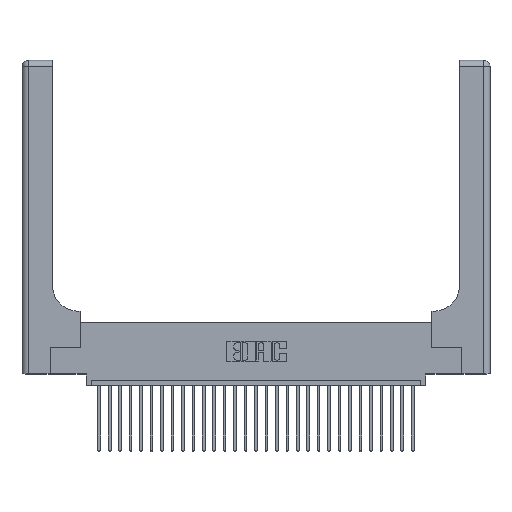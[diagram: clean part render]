
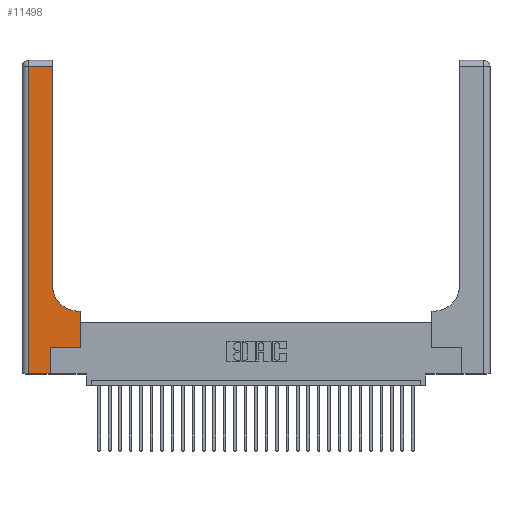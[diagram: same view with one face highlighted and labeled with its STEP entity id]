
A CAD part, top view. The second image highlights one B-rep face of the part: STEP entity #11498.
In plain terms, the highlighted planar face has unit normal (0, 0, 1).
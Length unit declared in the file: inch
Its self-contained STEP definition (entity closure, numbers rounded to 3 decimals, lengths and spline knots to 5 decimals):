
#89 = CARTESIAN_POINT ( 'NONE',  ( 0.5415, 0.6, 0.37 ) ) ;
#427 = CARTESIAN_POINT ( 'NONE',  ( 0.06, 3., 0.37 ) ) ;
#664 = LINE ( 'NONE', #8001, #13792 ) ;
#753 = LINE ( 'NONE', #427, #4031 ) ;
#1092 = DIRECTION ( 'NONE',  ( 1., 0., 0. ) ) ;
#1277 = VERTEX_POINT ( 'NONE', #27150 ) ;
#1534 = CARTESIAN_POINT ( 'NONE',  ( 0., 0., 0.37 ) ) ;
#1841 = DIRECTION ( 'NONE',  ( 1., 0., 0. ) ) ;
#2585 = DIRECTION ( 'NONE',  ( -1., 0., 0. ) ) ;
#2688 = CARTESIAN_POINT ( 'NONE',  ( 0., 3., 0.37 ) ) ;
#2798 = DIRECTION ( 'NONE',  ( 0., -1., 0. ) ) ;
#4031 = VECTOR ( 'NONE', #2798, 39.37008 ) ;
#4500 = CARTESIAN_POINT ( 'NONE',  ( 0., 2.94, 0.37 ) ) ;
#4639 = ORIENTED_EDGE ( 'NONE', *, *, #14295, .T. ) ;
#5188 = CARTESIAN_POINT ( 'NONE',  ( 0.2915, 3., 0.37 ) ) ;
#5705 = VERTEX_POINT ( 'NONE', #14656 ) ;
#5774 = FACE_OUTER_BOUND ( 'NONE', #26763, .T. ) ;
#5904 = VECTOR ( 'NONE', #29011, 39.37008 ) ;
#6970 = VECTOR ( 'NONE', #22443, 39.37008 ) ;
#7249 = CARTESIAN_POINT ( 'NONE',  ( 0.269, 0.25, 0.37 ) ) ;
#7587 = ORIENTED_EDGE ( 'NONE', *, *, #23187, .T. ) ;
#7790 = DIRECTION ( 'NONE',  ( 0., 1., 0. ) ) ;
#8001 = CARTESIAN_POINT ( 'NONE',  ( 0.5585, 0.25, 0.37 ) ) ;
#8144 = EDGE_CURVE ( 'NONE', #1277, #19769, #18276, .T. ) ;
#9527 = ORIENTED_EDGE ( 'NONE', *, *, #21666, .T. ) ;
#9698 = DIRECTION ( 'NONE',  ( 0., 0., -1. ) ) ;
#10090 = CIRCLE ( 'NONE', #21996, 0.25 ) ;
#10268 = LINE ( 'NONE', #26581, #5904 ) ;
#11498 = ADVANCED_FACE ( 'NONE', ( #5774 ), #18615, .F. ) ;
#11927 = DIRECTION ( 'NONE',  ( -1., 0., 0. ) ) ;
#12218 = EDGE_CURVE ( 'NONE', #16540, #15995, #20226, .T. ) ;
#13783 = EDGE_CURVE ( 'NONE', #5705, #16540, #10268, .T. ) ;
#13792 = VECTOR ( 'NONE', #7790, 39.37008 ) ;
#14163 = VECTOR ( 'NONE', #20651, 39.37008 ) ;
#14295 = EDGE_CURVE ( 'NONE', #17094, #5705, #20736, .T. ) ;
#14656 = CARTESIAN_POINT ( 'NONE',  ( 0.269, 0., 0.37 ) ) ;
#14816 = DIRECTION ( 'NONE',  ( 0., 1., 0. ) ) ;
#15369 = ORIENTED_EDGE ( 'NONE', *, *, #15416, .T. ) ;
#15416 = EDGE_CURVE ( 'NONE', #15532, #16965, #28680, .T. ) ;
#15532 = VERTEX_POINT ( 'NONE', #27781 ) ;
#15880 = VECTOR ( 'NONE', #1841, 39.37008 ) ;
#15995 = VERTEX_POINT ( 'NONE', #27072 ) ;
#16064 = ORIENTED_EDGE ( 'NONE', *, *, #13783, .T. ) ;
#16113 = AXIS2_PLACEMENT_3D ( 'NONE', #2688, #9698, #2585 ) ;
#16540 = VERTEX_POINT ( 'NONE', #7249 ) ;
#16965 = VERTEX_POINT ( 'NONE', #89 ) ;
#16997 = ORIENTED_EDGE ( 'NONE', *, *, #27641, .T. ) ;
#17094 = VERTEX_POINT ( 'NONE', #28500 ) ;
#17261 = VERTEX_POINT ( 'NONE', #19739 ) ;
#17559 = ORIENTED_EDGE ( 'NONE', *, *, #12218, .T. ) ;
#18276 = LINE ( 'NONE', #5188, #27735 ) ;
#18615 = PLANE ( 'NONE',  #16113 ) ;
#18823 = VECTOR ( 'NONE', #11927, 39.37008 ) ;
#19739 = CARTESIAN_POINT ( 'NONE',  ( 0.06, 2.94, 0.37 ) ) ;
#19769 = VERTEX_POINT ( 'NONE', #29572 ) ;
#20226 = LINE ( 'NONE', #20386, #15880 ) ;
#20386 = CARTESIAN_POINT ( 'NONE',  ( 0.269, 0.25, 0.37 ) ) ;
#20651 = DIRECTION ( 'NONE',  ( -1., 0., 0. ) ) ;
#20736 = LINE ( 'NONE', #1534, #6970 ) ;
#21592 = ORIENTED_EDGE ( 'NONE', *, *, #22964, .T. ) ;
#21666 = EDGE_CURVE ( 'NONE', #17261, #17094, #753, .T. ) ;
#21797 = DIRECTION ( 'NONE',  ( 0., 0., -1. ) ) ;
#21996 = AXIS2_PLACEMENT_3D ( 'NONE', #26803, #21797, #1092 ) ;
#22443 = DIRECTION ( 'NONE',  ( 1., 0., 0. ) ) ;
#22964 = EDGE_CURVE ( 'NONE', #15995, #15532, #664, .T. ) ;
#23187 = EDGE_CURVE ( 'NONE', #19769, #17261, #25024, .T. ) ;
#23608 = ORIENTED_EDGE ( 'NONE', *, *, #8144, .T. ) ;
#25024 = LINE ( 'NONE', #4500, #18823 ) ;
#26581 = CARTESIAN_POINT ( 'NONE',  ( 0.269, 0., 0.37 ) ) ;
#26763 = EDGE_LOOP ( 'NONE', ( #23608, #7587, #9527, #4639, #16064, #17559, #21592, #15369, #16997 ) ) ;
#26803 = CARTESIAN_POINT ( 'NONE',  ( 0.5415, 0.85, 0.37 ) ) ;
#27072 = CARTESIAN_POINT ( 'NONE',  ( 0.5585, 0.25, 0.37 ) ) ;
#27150 = CARTESIAN_POINT ( 'NONE',  ( 0.2915, 0.85, 0.37 ) ) ;
#27641 = EDGE_CURVE ( 'NONE', #16965, #1277, #10090, .T. ) ;
#27735 = VECTOR ( 'NONE', #14816, 39.37008 ) ;
#27781 = CARTESIAN_POINT ( 'NONE',  ( 0.5585, 0.6, 0.37 ) ) ;
#28500 = CARTESIAN_POINT ( 'NONE',  ( 0.06, 0., 0.37 ) ) ;
#28680 = LINE ( 'NONE', #29941, #14163 ) ;
#29011 = DIRECTION ( 'NONE',  ( 0., 1., 0. ) ) ;
#29572 = CARTESIAN_POINT ( 'NONE',  ( 0.2915, 2.94, 0.37 ) ) ;
#29941 = CARTESIAN_POINT ( 'NONE',  ( 0.2915, 0.6, 0.37 ) ) ;
